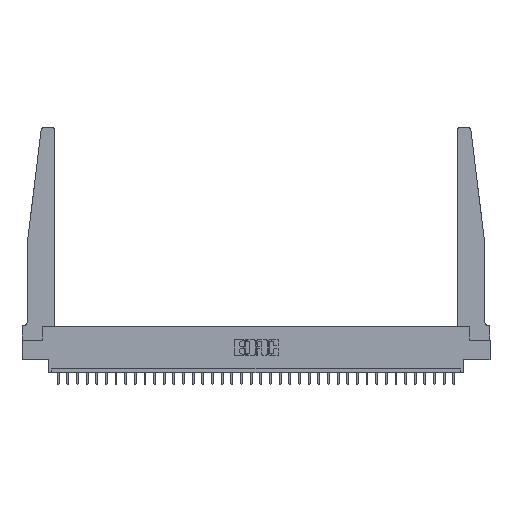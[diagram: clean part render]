
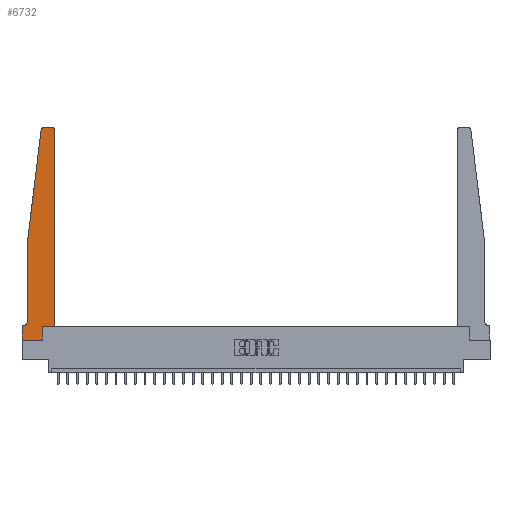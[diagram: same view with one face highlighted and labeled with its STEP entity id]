
A CAD part, top view. The second image highlights one B-rep face of the part: STEP entity #6732.
In plain terms, the highlighted planar face has unit normal (0, 0, 1).
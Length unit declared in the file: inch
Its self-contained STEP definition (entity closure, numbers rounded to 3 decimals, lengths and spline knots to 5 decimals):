
#117 = ORIENTED_EDGE ( 'NONE', *, *, #15879, .T. ) ;
#308 = LINE ( 'NONE', #27801, #7730 ) ;
#349 = CARTESIAN_POINT ( 'NONE',  ( 0.24675, 2.72367, 0.37 ) ) ;
#613 = DIRECTION ( 'NONE',  ( 0., 0., -1. ) ) ;
#624 = LINE ( 'NONE', #2374, #30524 ) ;
#880 = EDGE_CURVE ( 'NONE', #6363, #24562, #308, .T. ) ;
#1298 = AXIS2_PLACEMENT_3D ( 'NONE', #14688, #613, #24326 ) ;
#2006 = VECTOR ( 'NONE', #20002, 39.37008 ) ;
#2098 = DIRECTION ( 'NONE',  ( 0., 0., 1. ) ) ;
#2374 = CARTESIAN_POINT ( 'NONE',  ( 0.25, 2.75, 0.37 ) ) ;
#2422 = VECTOR ( 'NONE', #17454, 39.37008 ) ;
#2437 = CARTESIAN_POINT ( 'NONE',  ( 0., 0., 0.37 ) ) ;
#2584 = EDGE_CURVE ( 'NONE', #4742, #10210, #624, .T. ) ;
#2760 = DIRECTION ( 'NONE',  ( 1., 0., 0. ) ) ;
#3685 = LINE ( 'NONE', #28739, #16091 ) ;
#4103 = FACE_OUTER_BOUND ( 'NONE', #14046, .T. ) ;
#4282 = DIRECTION ( 'NONE',  ( -0.122, -0.992, 0. ) ) ;
#4374 = VECTOR ( 'NONE', #27232, 39.37008 ) ;
#4475 = DIRECTION ( 'NONE',  ( 1., 0., 0. ) ) ;
#4742 = VERTEX_POINT ( 'NONE', #22596 ) ;
#5061 = VERTEX_POINT ( 'NONE', #349 ) ;
#5111 = CARTESIAN_POINT ( 'NONE',  ( 0.065, 1.25, 0.37 ) ) ;
#5134 = VECTOR ( 'NONE', #19586, 39.37008 ) ;
#5615 = VERTEX_POINT ( 'NONE', #22092 ) ;
#6265 = LINE ( 'NONE', #20156, #4374 ) ;
#6363 = VERTEX_POINT ( 'NONE', #30930 ) ;
#6732 = ADVANCED_FACE ( 'NONE', ( #4103 ), #16500, .T. ) ;
#7730 = VECTOR ( 'NONE', #21036, 39.37008 ) ;
#7809 = EDGE_CURVE ( 'NONE', #29911, #20571, #23495, .T. ) ;
#9083 = CARTESIAN_POINT ( 'NONE',  ( 0., 0.1875, 0.37 ) ) ;
#9755 = CIRCLE ( 'NONE', #10038, 0.03 ) ;
#9936 = EDGE_CURVE ( 'NONE', #20571, #30307, #21106, .T. ) ;
#10038 = AXIS2_PLACEMENT_3D ( 'NONE', #22558, #10613, #27351 ) ;
#10210 = VERTEX_POINT ( 'NONE', #17528 ) ;
#10613 = DIRECTION ( 'NONE',  ( 0., 0., 1. ) ) ;
#10662 = CARTESIAN_POINT ( 'NONE',  ( 0.2605, 0.18, 0.37 ) ) ;
#12039 = ORIENTED_EDGE ( 'NONE', *, *, #7809, .T. ) ;
#12184 = ORIENTED_EDGE ( 'NONE', *, *, #30966, .T. ) ;
#12628 = EDGE_CURVE ( 'NONE', #5061, #30126, #14123, .T. ) ;
#12818 = ORIENTED_EDGE ( 'NONE', *, *, #2584, .T. ) ;
#14046 = EDGE_LOOP ( 'NONE', ( #12818, #12184, #16118, #117, #30443, #16571, #16437, #26578, #12039, #19646, #19840, #22640 ) ) ;
#14123 = LINE ( 'NONE', #30080, #23884 ) ;
#14182 = AXIS2_PLACEMENT_3D ( 'NONE', #9083, #2098, #4475 ) ;
#14592 = CARTESIAN_POINT ( 'NONE',  ( 0.27653, 2.72, 0.37 ) ) ;
#14688 = CARTESIAN_POINT ( 'NONE',  ( 0.015, 0.2375, 0.37 ) ) ;
#15016 = DIRECTION ( 'NONE',  ( 1., 0., 0. ) ) ;
#15096 = DIRECTION ( 'NONE',  ( -1., 0., 0. ) ) ;
#15879 = EDGE_CURVE ( 'NONE', #30126, #5615, #28985, .T. ) ;
#16091 = VECTOR ( 'NONE', #21221, 39.37008 ) ;
#16118 = ORIENTED_EDGE ( 'NONE', *, *, #12628, .T. ) ;
#16437 = ORIENTED_EDGE ( 'NONE', *, *, #28662, .T. ) ;
#16500 = PLANE ( 'NONE',  #14182 ) ;
#16571 = ORIENTED_EDGE ( 'NONE', *, *, #880, .T. ) ;
#17454 = DIRECTION ( 'NONE',  ( 0., -1., 0. ) ) ;
#17528 = CARTESIAN_POINT ( 'NONE',  ( 0.27653, 2.75, 0.37 ) ) ;
#19267 = CARTESIAN_POINT ( 'NONE',  ( 0.425, 0.18, 0.37 ) ) ;
#19586 = DIRECTION ( 'NONE',  ( 0., 1., 0. ) ) ;
#19646 = ORIENTED_EDGE ( 'NONE', *, *, #9936, .T. ) ;
#19763 = DIRECTION ( 'NONE',  ( 0., 0., 1. ) ) ;
#19840 = ORIENTED_EDGE ( 'NONE', *, *, #23984, .T. ) ;
#20002 = DIRECTION ( 'NONE',  ( 1., 0., 0. ) ) ;
#20097 = CARTESIAN_POINT ( 'NONE',  ( 0.425, 0.18, 0.37 ) ) ;
#20156 = CARTESIAN_POINT ( 'NONE',  ( 0.425, 0.18, 0.37 ) ) ;
#20571 = VERTEX_POINT ( 'NONE', #10662 ) ;
#20727 = VECTOR ( 'NONE', #2760, 39.37008 ) ;
#20731 = VERTEX_POINT ( 'NONE', #2437 ) ;
#20846 = AXIS2_PLACEMENT_3D ( 'NONE', #14592, #19763, #15016 ) ;
#21036 = DIRECTION ( 'NONE',  ( -1., 0., 0. ) ) ;
#21106 = LINE ( 'NONE', #20097, #2006 ) ;
#21221 = DIRECTION ( 'NONE',  ( 0., -1., 0. ) ) ;
#21336 = VERTEX_POINT ( 'NONE', #24040 ) ;
#21991 = CIRCLE ( 'NONE', #1298, 0.05 ) ;
#22092 = CARTESIAN_POINT ( 'NONE',  ( 0.065, 0.2375, 0.37 ) ) ;
#22532 = EDGE_CURVE ( 'NONE', #21336, #4742, #9755, .T. ) ;
#22558 = CARTESIAN_POINT ( 'NONE',  ( 0.395, 2.72, 0.37 ) ) ;
#22596 = CARTESIAN_POINT ( 'NONE',  ( 0.395, 2.75, 0.37 ) ) ;
#22640 = ORIENTED_EDGE ( 'NONE', *, *, #22532, .T. ) ;
#23495 = LINE ( 'NONE', #28680, #5134 ) ;
#23884 = VECTOR ( 'NONE', #4282, 39.37008 ) ;
#23984 = EDGE_CURVE ( 'NONE', #30307, #21336, #6265, .T. ) ;
#24040 = CARTESIAN_POINT ( 'NONE',  ( 0.425, 2.72, 0.37 ) ) ;
#24215 = EDGE_CURVE ( 'NONE', #5615, #6363, #21991, .T. ) ;
#24326 = DIRECTION ( 'NONE',  ( -1., 0., 0. ) ) ;
#24562 = VERTEX_POINT ( 'NONE', #28280 ) ;
#26052 = CARTESIAN_POINT ( 'NONE',  ( 0.065, 1.25, 0.37 ) ) ;
#26562 = EDGE_CURVE ( 'NONE', #20731, #29911, #28570, .T. ) ;
#26578 = ORIENTED_EDGE ( 'NONE', *, *, #26562, .T. ) ;
#27232 = DIRECTION ( 'NONE',  ( 0., 1., 0. ) ) ;
#27351 = DIRECTION ( 'NONE',  ( 1., 0., 0. ) ) ;
#27519 = CIRCLE ( 'NONE', #20846, 0.03 ) ;
#27801 = CARTESIAN_POINT ( 'NONE',  ( 0.065, 0.1875, 0.37 ) ) ;
#28280 = CARTESIAN_POINT ( 'NONE',  ( 0., 0.1875, 0.37 ) ) ;
#28408 = CARTESIAN_POINT ( 'NONE',  ( 0., 0., 0.37 ) ) ;
#28570 = LINE ( 'NONE', #28408, #20727 ) ;
#28662 = EDGE_CURVE ( 'NONE', #24562, #20731, #3685, .T. ) ;
#28680 = CARTESIAN_POINT ( 'NONE',  ( 0.2605, 0.18, 0.37 ) ) ;
#28739 = CARTESIAN_POINT ( 'NONE',  ( 0., 0., 0.37 ) ) ;
#28985 = LINE ( 'NONE', #5111, #2422 ) ;
#29911 = VERTEX_POINT ( 'NONE', #30185 ) ;
#30080 = CARTESIAN_POINT ( 'NONE',  ( 0.065, 1.25, 0.37 ) ) ;
#30126 = VERTEX_POINT ( 'NONE', #26052 ) ;
#30185 = CARTESIAN_POINT ( 'NONE',  ( 0.2605, 0., 0.37 ) ) ;
#30307 = VERTEX_POINT ( 'NONE', #19267 ) ;
#30443 = ORIENTED_EDGE ( 'NONE', *, *, #24215, .T. ) ;
#30524 = VECTOR ( 'NONE', #15096, 39.37008 ) ;
#30930 = CARTESIAN_POINT ( 'NONE',  ( 0.015, 0.1875, 0.37 ) ) ;
#30966 = EDGE_CURVE ( 'NONE', #10210, #5061, #27519, .T. ) ;
